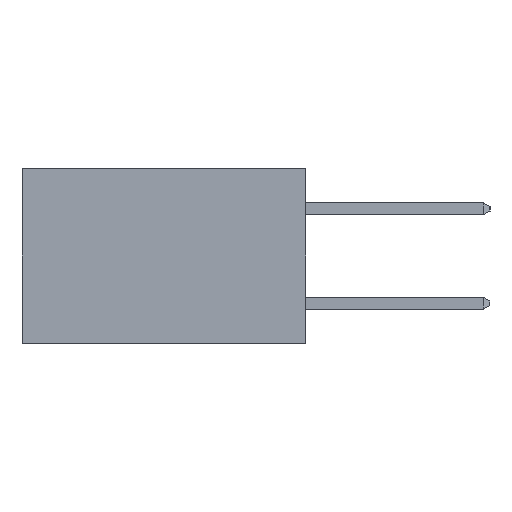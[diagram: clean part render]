
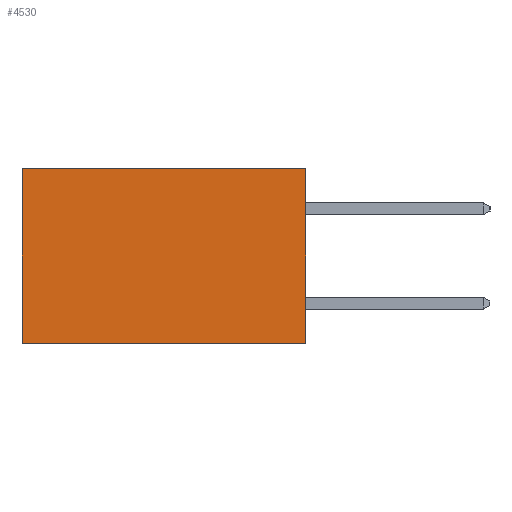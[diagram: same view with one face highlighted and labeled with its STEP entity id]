
A CAD part, left-side view. The second image highlights one B-rep face of the part: STEP entity #4530.
In plain terms, the highlighted planar face has unit normal (-1, 0, 0).
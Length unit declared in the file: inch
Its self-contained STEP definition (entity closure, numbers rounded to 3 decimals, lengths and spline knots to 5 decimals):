
#399 = CARTESIAN_POINT ( 'NONE',  ( 0.298, 0., 0. ) ) ;
#1273 = EDGE_LOOP ( 'NONE', ( #14183, #6774, #3601, #7701 ) ) ;
#1452 = VERTEX_POINT ( 'NONE', #11807 ) ;
#1460 = LINE ( 'NONE', #14367, #16982 ) ;
#1556 = DIRECTION ( 'NONE',  ( 0., 1., 0. ) ) ;
#1843 = EDGE_CURVE ( 'NONE', #5726, #1452, #14737, .T. ) ;
#2644 = VERTEX_POINT ( 'NONE', #9392 ) ;
#3569 = DIRECTION ( 'NONE',  ( 0., 0., -1. ) ) ;
#3601 = ORIENTED_EDGE ( 'NONE', *, *, #4424, .F. ) ;
#4144 = VECTOR ( 'NONE', #16044, 39.37008 ) ;
#4363 = EDGE_CURVE ( 'NONE', #2644, #1452, #1460, .T. ) ;
#4424 = EDGE_CURVE ( 'NONE', #17446, #5726, #12026, .T. ) ;
#4530 = ADVANCED_FACE ( 'NONE', ( #9695 ), #18207, .F. ) ;
#5726 = VERTEX_POINT ( 'NONE', #16961 ) ;
#6244 = AXIS2_PLACEMENT_3D ( 'NONE', #8878, #18271, #3569 ) ;
#6752 = VECTOR ( 'NONE', #1556, 39.37008 ) ;
#6774 = ORIENTED_EDGE ( 'NONE', *, *, #1843, .F. ) ;
#7701 = ORIENTED_EDGE ( 'NONE', *, *, #16181, .T. ) ;
#8878 = CARTESIAN_POINT ( 'NONE',  ( 0.298, 0., 0. ) ) ;
#9392 = CARTESIAN_POINT ( 'NONE',  ( 0.298, 0.6, 0. ) ) ;
#9695 = FACE_OUTER_BOUND ( 'NONE', #1273, .T. ) ;
#9762 = DIRECTION ( 'NONE',  ( 0., 0., -1. ) ) ;
#11142 = CARTESIAN_POINT ( 'NONE',  ( 0.298, 0., -0.37 ) ) ;
#11807 = CARTESIAN_POINT ( 'NONE',  ( 0.298, 0.6, -0.37 ) ) ;
#12026 = LINE ( 'NONE', #15985, #4144 ) ;
#12420 = CARTESIAN_POINT ( 'NONE',  ( 0.298, 0., 0. ) ) ;
#13847 = DIRECTION ( 'NONE',  ( 0., 1., 0. ) ) ;
#14183 = ORIENTED_EDGE ( 'NONE', *, *, #4363, .T. ) ;
#14367 = CARTESIAN_POINT ( 'NONE',  ( 0.298, 0.6, 0. ) ) ;
#14737 = LINE ( 'NONE', #11142, #6752 ) ;
#15985 = CARTESIAN_POINT ( 'NONE',  ( 0.298, 0., 0. ) ) ;
#16044 = DIRECTION ( 'NONE',  ( 0., 0., -1. ) ) ;
#16181 = EDGE_CURVE ( 'NONE', #17446, #2644, #18900, .T. ) ;
#16961 = CARTESIAN_POINT ( 'NONE',  ( 0.298, 0., -0.37 ) ) ;
#16982 = VECTOR ( 'NONE', #9762, 39.37008 ) ;
#17446 = VERTEX_POINT ( 'NONE', #12420 ) ;
#18207 = PLANE ( 'NONE',  #6244 ) ;
#18271 = DIRECTION ( 'NONE',  ( 1., 0., 0. ) ) ;
#18443 = VECTOR ( 'NONE', #13847, 39.37008 ) ;
#18900 = LINE ( 'NONE', #399, #18443 ) ;
